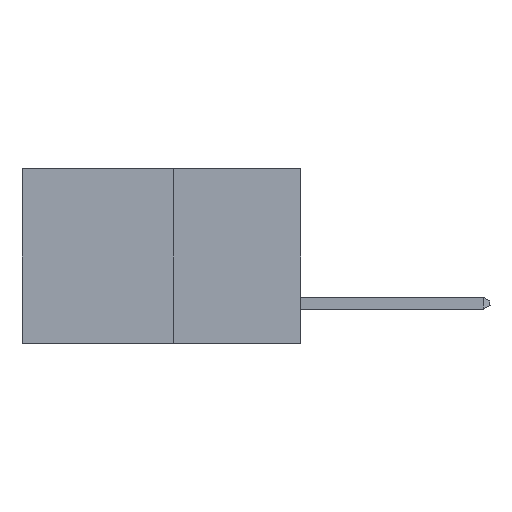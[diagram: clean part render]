
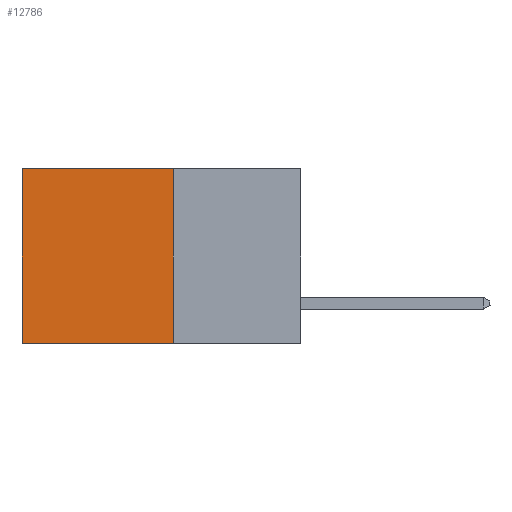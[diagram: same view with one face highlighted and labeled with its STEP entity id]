
A CAD part, left-side view. The second image highlights one B-rep face of the part: STEP entity #12786.
In plain terms, the highlighted planar face has unit normal (-1, 0, 0).
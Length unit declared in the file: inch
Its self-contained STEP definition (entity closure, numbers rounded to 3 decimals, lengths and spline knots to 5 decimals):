
#137 = DIRECTION ( 'NONE',  ( 0., 0., -1. ) ) ;
#233 = CARTESIAN_POINT ( 'NONE',  ( 0.277, 0.27, 0. ) ) ;
#328 = VECTOR ( 'NONE', #10291, 39.37008 ) ;
#465 = VERTEX_POINT ( 'NONE', #6576 ) ;
#472 = DIRECTION ( 'NONE',  ( 1., 0., 0. ) ) ;
#684 = EDGE_LOOP ( 'NONE', ( #18538, #9517, #17461, #6448 ) ) ;
#1166 = CARTESIAN_POINT ( 'NONE',  ( 0.277, 0.27, -0.37 ) ) ;
#2205 = VECTOR ( 'NONE', #8467, 39.37008 ) ;
#3413 = LINE ( 'NONE', #4691, #11038 ) ;
#3520 = CARTESIAN_POINT ( 'NONE',  ( 0.277, 0.27, -0.37 ) ) ;
#4691 = CARTESIAN_POINT ( 'NONE',  ( 0.277, 0.59, -0.37 ) ) ;
#4782 = VERTEX_POINT ( 'NONE', #233 ) ;
#4877 = LINE ( 'NONE', #1166, #328 ) ;
#6448 = ORIENTED_EDGE ( 'NONE', *, *, #9030, .T. ) ;
#6576 = CARTESIAN_POINT ( 'NONE',  ( 0.277, 0.59, -0.37 ) ) ;
#6578 = CARTESIAN_POINT ( 'NONE',  ( 0.277, 0.27, -0.37 ) ) ;
#7687 = VECTOR ( 'NONE', #9637, 39.37008 ) ;
#8467 = DIRECTION ( 'NONE',  ( 0., 1., 0. ) ) ;
#9030 = EDGE_CURVE ( 'NONE', #4782, #16580, #10318, .T. ) ;
#9207 = CARTESIAN_POINT ( 'NONE',  ( 0.277, 0.59, 0. ) ) ;
#9517 = ORIENTED_EDGE ( 'NONE', *, *, #10063, .F. ) ;
#9637 = DIRECTION ( 'NONE',  ( 0., 1., 0. ) ) ;
#10063 = EDGE_CURVE ( 'NONE', #10076, #465, #11737, .T. ) ;
#10076 = VERTEX_POINT ( 'NONE', #17128 ) ;
#10291 = DIRECTION ( 'NONE',  ( 0., 0., -1. ) ) ;
#10318 = LINE ( 'NONE', #14572, #2205 ) ;
#11038 = VECTOR ( 'NONE', #137, 39.37008 ) ;
#11152 = DIRECTION ( 'NONE',  ( 0., 0., -1. ) ) ;
#11737 = LINE ( 'NONE', #3520, #7687 ) ;
#12554 = EDGE_CURVE ( 'NONE', #4782, #10076, #4877, .T. ) ;
#12786 = ADVANCED_FACE ( 'NONE', ( #19193 ), #15629, .F. ) ;
#14572 = CARTESIAN_POINT ( 'NONE',  ( 0.277, 0.27, 0. ) ) ;
#15629 = PLANE ( 'NONE',  #19163 ) ;
#16580 = VERTEX_POINT ( 'NONE', #9207 ) ;
#17128 = CARTESIAN_POINT ( 'NONE',  ( 0.277, 0.27, -0.37 ) ) ;
#17461 = ORIENTED_EDGE ( 'NONE', *, *, #12554, .F. ) ;
#18020 = EDGE_CURVE ( 'NONE', #16580, #465, #3413, .T. ) ;
#18538 = ORIENTED_EDGE ( 'NONE', *, *, #18020, .T. ) ;
#19163 = AXIS2_PLACEMENT_3D ( 'NONE', #6578, #472, #11152 ) ;
#19193 = FACE_OUTER_BOUND ( 'NONE', #684, .T. ) ;
